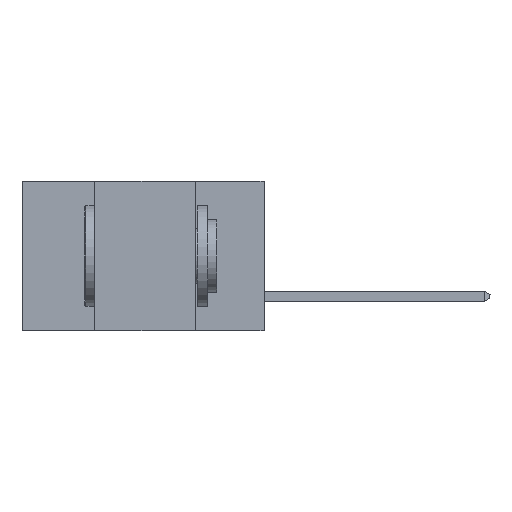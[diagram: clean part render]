
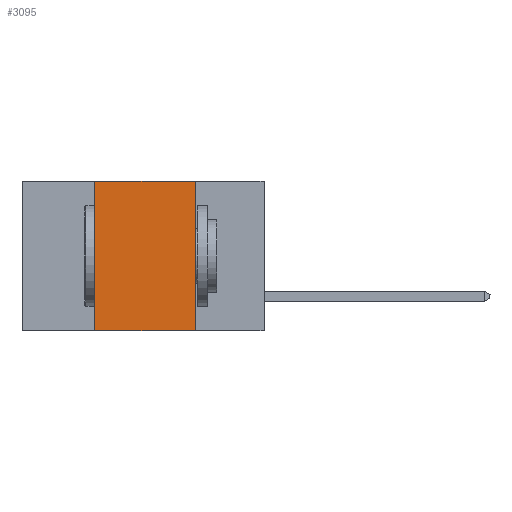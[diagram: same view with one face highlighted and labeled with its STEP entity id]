
A CAD part, left-side view. The second image highlights one B-rep face of the part: STEP entity #3095.
In plain terms, the highlighted planar face has unit normal (-1, 0, 0).
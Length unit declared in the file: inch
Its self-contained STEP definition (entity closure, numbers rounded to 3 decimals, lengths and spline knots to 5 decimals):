
#101 = LINE ( 'NONE', #18190, #5472 ) ;
#368 = VERTEX_POINT ( 'NONE', #1269 ) ;
#689 = DIRECTION ( 'NONE',  ( 0., 0., -1. ) ) ;
#1269 = CARTESIAN_POINT ( 'NONE',  ( 0., 0.42, 0. ) ) ;
#1431 = CARTESIAN_POINT ( 'NONE',  ( 0., 0.42, 0. ) ) ;
#2155 = VECTOR ( 'NONE', #26459, 39.37008 ) ;
#2305 = VECTOR ( 'NONE', #3572, 39.37008 ) ;
#2370 = EDGE_CURVE ( 'NONE', #25248, #27513, #5191, .T. ) ;
#2891 = AXIS2_PLACEMENT_3D ( 'NONE', #3032, #22338, #689 ) ;
#3032 = CARTESIAN_POINT ( 'NONE',  ( 0., 0.6, 0. ) ) ;
#3095 = ADVANCED_FACE ( 'NONE', ( #3136 ), #15870, .F. ) ;
#3136 = FACE_OUTER_BOUND ( 'NONE', #23484, .T. ) ;
#3222 = CARTESIAN_POINT ( 'NONE',  ( 0., 0.6, -0.37 ) ) ;
#3572 = DIRECTION ( 'NONE',  ( 0., 0., 1. ) ) ;
#3992 = CARTESIAN_POINT ( 'NONE',  ( 0., 0.17, -0.37 ) ) ;
#5191 = LINE ( 'NONE', #3222, #20595 ) ;
#5472 = VECTOR ( 'NONE', #5524, 39.37008 ) ;
#5524 = DIRECTION ( 'NONE',  ( 0., 0., -1. ) ) ;
#6112 = EDGE_CURVE ( 'NONE', #25248, #368, #19750, .T. ) ;
#11407 = CARTESIAN_POINT ( 'NONE',  ( 0., 0.42, -0.37 ) ) ;
#13875 = LINE ( 'NONE', #15619, #2155 ) ;
#15113 = ORIENTED_EDGE ( 'NONE', *, *, #2370, .T. ) ;
#15619 = CARTESIAN_POINT ( 'NONE',  ( 0., 0.6, 0. ) ) ;
#15870 = PLANE ( 'NONE',  #2891 ) ;
#16248 = DIRECTION ( 'NONE',  ( 0., -1., 0. ) ) ;
#18049 = ORIENTED_EDGE ( 'NONE', *, *, #19092, .F. ) ;
#18190 = CARTESIAN_POINT ( 'NONE',  ( 0., 0.17, 0. ) ) ;
#19092 = EDGE_CURVE ( 'NONE', #368, #22778, #13875, .T. ) ;
#19750 = LINE ( 'NONE', #1431, #2305 ) ;
#20595 = VECTOR ( 'NONE', #16248, 39.37008 ) ;
#20785 = ORIENTED_EDGE ( 'NONE', *, *, #26932, .F. ) ;
#22338 = DIRECTION ( 'NONE',  ( 1., 0., 0. ) ) ;
#22610 = ORIENTED_EDGE ( 'NONE', *, *, #6112, .F. ) ;
#22778 = VERTEX_POINT ( 'NONE', #25182 ) ;
#23484 = EDGE_LOOP ( 'NONE', ( #20785, #18049, #22610, #15113 ) ) ;
#25182 = CARTESIAN_POINT ( 'NONE',  ( 0., 0.17, 0. ) ) ;
#25248 = VERTEX_POINT ( 'NONE', #11407 ) ;
#26459 = DIRECTION ( 'NONE',  ( 0., -1., 0. ) ) ;
#26932 = EDGE_CURVE ( 'NONE', #22778, #27513, #101, .T. ) ;
#27513 = VERTEX_POINT ( 'NONE', #3992 ) ;
